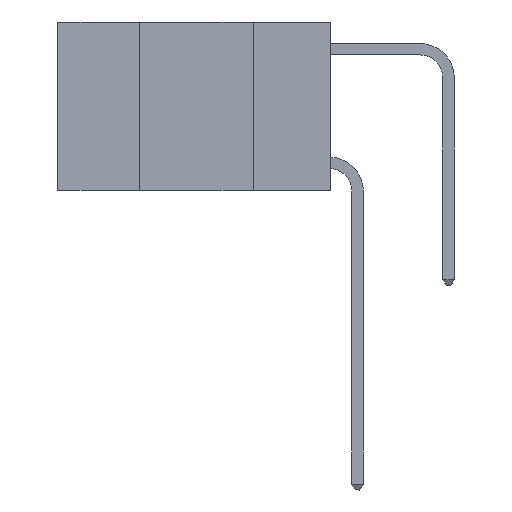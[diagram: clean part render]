
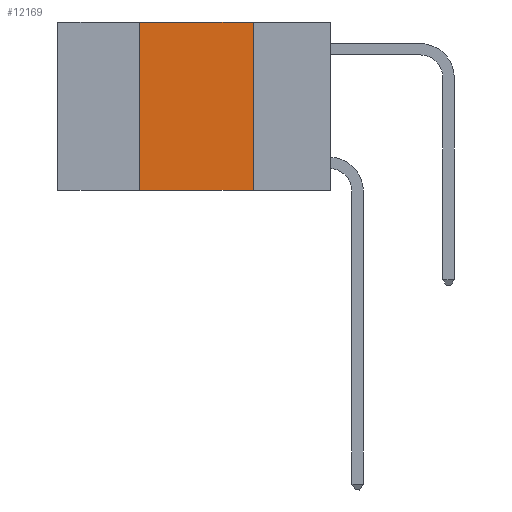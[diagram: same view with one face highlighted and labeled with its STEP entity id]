
A CAD part, left-side view. The second image highlights one B-rep face of the part: STEP entity #12169.
In plain terms, the highlighted planar face has unit normal (-1, 0, 0).
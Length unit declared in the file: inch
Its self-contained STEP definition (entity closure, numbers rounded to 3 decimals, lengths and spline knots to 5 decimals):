
#584 = LINE ( 'NONE', #11068, #9235 ) ;
#1148 = ORIENTED_EDGE ( 'NONE', *, *, #9603, .F. ) ;
#1176 = ORIENTED_EDGE ( 'NONE', *, *, #11838, .F. ) ;
#1275 = ORIENTED_EDGE ( 'NONE', *, *, #10649, .F. ) ;
#1291 = ORIENTED_EDGE ( 'NONE', *, *, #2883, .T. ) ;
#1504 = EDGE_LOOP ( 'NONE', ( #1148, #1176, #1275, #1291 ) ) ;
#1921 = VERTEX_POINT ( 'NONE', #11326 ) ;
#2040 = LINE ( 'NONE', #11740, #7670 ) ;
#2883 = EDGE_CURVE ( 'NONE', #5029, #5250, #13258, .T. ) ;
#3076 = CARTESIAN_POINT ( 'NONE',  ( 0., 0.17, -0.37 ) ) ;
#3282 = DIRECTION ( 'NONE',  ( 0., 0., 1. ) ) ;
#3481 = AXIS2_PLACEMENT_3D ( 'NONE', #11011, #14284, #7708 ) ;
#5029 = VERTEX_POINT ( 'NONE', #9388 ) ;
#5250 = VERTEX_POINT ( 'NONE', #3076 ) ;
#5684 = VERTEX_POINT ( 'NONE', #7132 ) ;
#6584 = PLANE ( 'NONE',  #3481 ) ;
#6740 = FACE_OUTER_BOUND ( 'NONE', #1504, .T. ) ;
#7019 = VECTOR ( 'NONE', #10915, 39.37008 ) ;
#7132 = CARTESIAN_POINT ( 'NONE',  ( 0., 0.42, 0. ) ) ;
#7506 = CARTESIAN_POINT ( 'NONE',  ( 0., 0.6, 0. ) ) ;
#7670 = VECTOR ( 'NONE', #12854, 39.37008 ) ;
#7708 = DIRECTION ( 'NONE',  ( 0., 0., -1. ) ) ;
#8703 = VECTOR ( 'NONE', #13089, 39.37008 ) ;
#8796 = CARTESIAN_POINT ( 'NONE',  ( 0., 0.6, -0.37 ) ) ;
#9235 = VECTOR ( 'NONE', #3282, 39.37008 ) ;
#9388 = CARTESIAN_POINT ( 'NONE',  ( 0., 0.42, -0.37 ) ) ;
#9603 = EDGE_CURVE ( 'NONE', #1921, #5250, #2040, .T. ) ;
#10649 = EDGE_CURVE ( 'NONE', #5029, #5684, #584, .T. ) ;
#10915 = DIRECTION ( 'NONE',  ( 0., -1., 0. ) ) ;
#11011 = CARTESIAN_POINT ( 'NONE',  ( 0., 0.6, 0. ) ) ;
#11068 = CARTESIAN_POINT ( 'NONE',  ( 0., 0.42, 0. ) ) ;
#11326 = CARTESIAN_POINT ( 'NONE',  ( 0., 0.17, 0. ) ) ;
#11624 = LINE ( 'NONE', #7506, #8703 ) ;
#11740 = CARTESIAN_POINT ( 'NONE',  ( 0., 0.17, 0. ) ) ;
#11838 = EDGE_CURVE ( 'NONE', #5684, #1921, #11624, .T. ) ;
#12169 = ADVANCED_FACE ( 'NONE', ( #6740 ), #6584, .F. ) ;
#12854 = DIRECTION ( 'NONE',  ( 0., 0., -1. ) ) ;
#13089 = DIRECTION ( 'NONE',  ( 0., -1., 0. ) ) ;
#13258 = LINE ( 'NONE', #8796, #7019 ) ;
#14284 = DIRECTION ( 'NONE',  ( 1., 0., 0. ) ) ;
